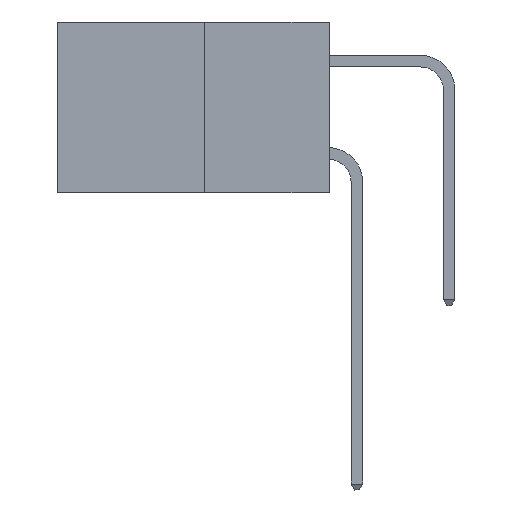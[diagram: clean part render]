
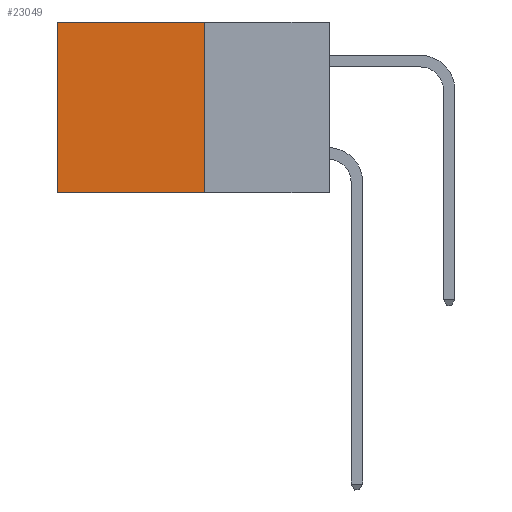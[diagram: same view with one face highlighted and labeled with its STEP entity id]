
A CAD part, left-side view. The second image highlights one B-rep face of the part: STEP entity #23049.
In plain terms, the highlighted planar face has unit normal (-1, 0, 0).
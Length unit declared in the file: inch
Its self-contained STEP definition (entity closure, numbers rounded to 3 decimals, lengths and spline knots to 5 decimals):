
#120 = DIRECTION ( 'NONE',  ( 1., 0., 0. ) ) ;
#750 = EDGE_CURVE ( 'NONE', #19198, #12592, #18796, .T. ) ;
#2389 = ORIENTED_EDGE ( 'NONE', *, *, #750, .F. ) ;
#2573 = CARTESIAN_POINT ( 'NONE',  ( 0.277, 0.27, 0. ) ) ;
#3100 = LINE ( 'NONE', #23120, #27838 ) ;
#4132 = EDGE_CURVE ( 'NONE', #31753, #19198, #3100, .T. ) ;
#7058 = CARTESIAN_POINT ( 'NONE',  ( 0.277, 0.59, -0.37 ) ) ;
#7289 = CARTESIAN_POINT ( 'NONE',  ( 0.277, 0.27, -0.37 ) ) ;
#7949 = VECTOR ( 'NONE', #24022, 39.37008 ) ;
#8796 = LINE ( 'NONE', #10937, #7949 ) ;
#10074 = AXIS2_PLACEMENT_3D ( 'NONE', #29095, #120, #18767 ) ;
#10937 = CARTESIAN_POINT ( 'NONE',  ( 0.277, 0.59, -0.37 ) ) ;
#12592 = VERTEX_POINT ( 'NONE', #7058 ) ;
#15379 = EDGE_CURVE ( 'NONE', #29105, #12592, #8796, .T. ) ;
#16108 = ORIENTED_EDGE ( 'NONE', *, *, #25614, .T. ) ;
#18640 = CARTESIAN_POINT ( 'NONE',  ( 0.277, 0.27, 0. ) ) ;
#18767 = DIRECTION ( 'NONE',  ( 0., 0., -1. ) ) ;
#18796 = LINE ( 'NONE', #31393, #24903 ) ;
#19198 = VERTEX_POINT ( 'NONE', #7289 ) ;
#19320 = VECTOR ( 'NONE', #23642, 39.37008 ) ;
#21727 = DIRECTION ( 'NONE',  ( 0., 0., -1. ) ) ;
#22365 = FACE_OUTER_BOUND ( 'NONE', #27545, .T. ) ;
#23049 = ADVANCED_FACE ( 'NONE', ( #22365 ), #31648, .F. ) ;
#23100 = ORIENTED_EDGE ( 'NONE', *, *, #15379, .T. ) ;
#23120 = CARTESIAN_POINT ( 'NONE',  ( 0.277, 0.27, -0.37 ) ) ;
#23575 = ORIENTED_EDGE ( 'NONE', *, *, #4132, .F. ) ;
#23642 = DIRECTION ( 'NONE',  ( 0., 1., 0. ) ) ;
#24022 = DIRECTION ( 'NONE',  ( 0., 0., -1. ) ) ;
#24903 = VECTOR ( 'NONE', #30954, 39.37008 ) ;
#25614 = EDGE_CURVE ( 'NONE', #31753, #29105, #33025, .T. ) ;
#27545 = EDGE_LOOP ( 'NONE', ( #23100, #2389, #23575, #16108 ) ) ;
#27838 = VECTOR ( 'NONE', #21727, 39.37008 ) ;
#29095 = CARTESIAN_POINT ( 'NONE',  ( 0.277, 0.27, -0.37 ) ) ;
#29105 = VERTEX_POINT ( 'NONE', #29458 ) ;
#29458 = CARTESIAN_POINT ( 'NONE',  ( 0.277, 0.59, 0. ) ) ;
#30954 = DIRECTION ( 'NONE',  ( 0., 1., 0. ) ) ;
#31393 = CARTESIAN_POINT ( 'NONE',  ( 0.277, 0.27, -0.37 ) ) ;
#31648 = PLANE ( 'NONE',  #10074 ) ;
#31753 = VERTEX_POINT ( 'NONE', #18640 ) ;
#33025 = LINE ( 'NONE', #2573, #19320 ) ;
